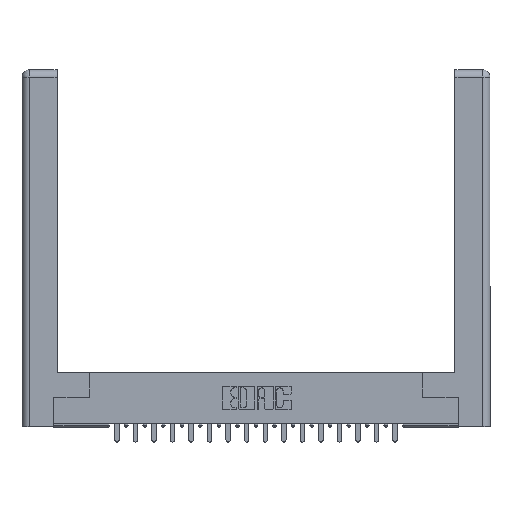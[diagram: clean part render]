
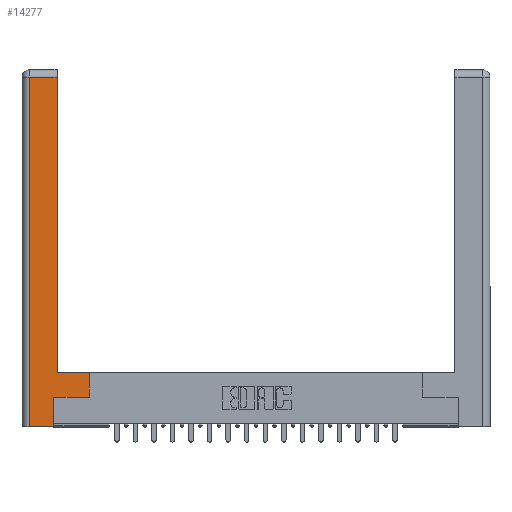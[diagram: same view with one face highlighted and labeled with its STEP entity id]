
A CAD part, top view. The second image highlights one B-rep face of the part: STEP entity #14277.
In plain terms, the highlighted planar face has unit normal (0, 0, 1).
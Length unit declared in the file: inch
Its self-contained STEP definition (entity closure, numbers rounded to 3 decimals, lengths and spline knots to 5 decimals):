
#419 = CARTESIAN_POINT ( 'NONE',  ( 0.265, 0.245, 0. ) ) ;
#942 = CARTESIAN_POINT ( 'NONE',  ( 0.565, 0.245, 0. ) ) ;
#1356 = EDGE_CURVE ( 'NONE', #6592, #10482, #18992, .T. ) ;
#1846 = CARTESIAN_POINT ( 'NONE',  ( 0.265, 0.245, 0. ) ) ;
#2085 = EDGE_CURVE ( 'NONE', #10482, #19898, #3635, .T. ) ;
#2226 = CARTESIAN_POINT ( 'NONE',  ( 0.295, 2.94, 0. ) ) ;
#2466 = ORIENTED_EDGE ( 'NONE', *, *, #19151, .T. ) ;
#2553 = VECTOR ( 'NONE', #2836, 39.37008 ) ;
#2600 = EDGE_CURVE ( 'NONE', #12772, #19252, #6533, .T. ) ;
#2634 = VECTOR ( 'NONE', #10267, 39.37008 ) ;
#2836 = DIRECTION ( 'NONE',  ( 1., 0., 0. ) ) ;
#3635 = LINE ( 'NONE', #16528, #2634 ) ;
#3648 = LINE ( 'NONE', #1846, #16045 ) ;
#4353 = VECTOR ( 'NONE', #9282, 39.37008 ) ;
#4514 = CARTESIAN_POINT ( 'NONE',  ( 0.295, 0.45, 0. ) ) ;
#4773 = DIRECTION ( 'NONE',  ( -1., 0., 0. ) ) ;
#4805 = ORIENTED_EDGE ( 'NONE', *, *, #6696, .T. ) ;
#5311 = ORIENTED_EDGE ( 'NONE', *, *, #2085, .T. ) ;
#6245 = DIRECTION ( 'NONE',  ( 0., 0., -1. ) ) ;
#6289 = EDGE_CURVE ( 'NONE', #19252, #18344, #16684, .T. ) ;
#6533 = LINE ( 'NONE', #16252, #16483 ) ;
#6592 = VERTEX_POINT ( 'NONE', #13665 ) ;
#6696 = EDGE_CURVE ( 'NONE', #19898, #12772, #10075, .T. ) ;
#7159 = AXIS2_PLACEMENT_3D ( 'NONE', #20623, #6245, #4773 ) ;
#7782 = ORIENTED_EDGE ( 'NONE', *, *, #1356, .T. ) ;
#8035 = VECTOR ( 'NONE', #19805, 39.37008 ) ;
#8288 = EDGE_LOOP ( 'NONE', ( #5311, #4805, #14075, #15988, #15586, #17774, #2466, #7782 ) ) ;
#9183 = LINE ( 'NONE', #942, #4353 ) ;
#9282 = DIRECTION ( 'NONE',  ( 1., 0., 0. ) ) ;
#9306 = PLANE ( 'NONE',  #7159 ) ;
#9372 = DIRECTION ( 'NONE',  ( -1., 0., 0. ) ) ;
#9645 = EDGE_CURVE ( 'NONE', #10732, #18544, #9183, .T. ) ;
#10075 = LINE ( 'NONE', #11977, #8035 ) ;
#10267 = DIRECTION ( 'NONE',  ( 0., 1., 0. ) ) ;
#10482 = VERTEX_POINT ( 'NONE', #12575 ) ;
#10528 = DIRECTION ( 'NONE',  ( 0., 1., 0. ) ) ;
#10629 = LINE ( 'NONE', #13599, #19137 ) ;
#10732 = VERTEX_POINT ( 'NONE', #419 ) ;
#10958 = DIRECTION ( 'NONE',  ( 0., -1., 0. ) ) ;
#11651 = VECTOR ( 'NONE', #9372, 39.37008 ) ;
#11977 = CARTESIAN_POINT ( 'NONE',  ( 0.0615, 2.94, 0. ) ) ;
#12575 = CARTESIAN_POINT ( 'NONE',  ( 0.295, 0.45, 0. ) ) ;
#12667 = CARTESIAN_POINT ( 'NONE',  ( 0.565, 0.245, 0. ) ) ;
#12772 = VERTEX_POINT ( 'NONE', #15934 ) ;
#13599 = CARTESIAN_POINT ( 'NONE',  ( 0.565, 0.45, 0. ) ) ;
#13665 = CARTESIAN_POINT ( 'NONE',  ( 0.565, 0.45, 0. ) ) ;
#13752 = CARTESIAN_POINT ( 'NONE',  ( 0.265, 0., 0. ) ) ;
#14075 = ORIENTED_EDGE ( 'NONE', *, *, #2600, .T. ) ;
#14277 = ADVANCED_FACE ( 'NONE', ( #19041 ), #9306, .F. ) ;
#15192 = CARTESIAN_POINT ( 'NONE',  ( 0.0615, 0., 0. ) ) ;
#15586 = ORIENTED_EDGE ( 'NONE', *, *, #17896, .T. ) ;
#15934 = CARTESIAN_POINT ( 'NONE',  ( 0.0615, 2.94, 0. ) ) ;
#15988 = ORIENTED_EDGE ( 'NONE', *, *, #6289, .T. ) ;
#16045 = VECTOR ( 'NONE', #19704, 39.37008 ) ;
#16252 = CARTESIAN_POINT ( 'NONE',  ( 0.0615, 0., 0. ) ) ;
#16483 = VECTOR ( 'NONE', #10958, 39.37008 ) ;
#16528 = CARTESIAN_POINT ( 'NONE',  ( 0.295, 3., 0. ) ) ;
#16684 = LINE ( 'NONE', #17001, #2553 ) ;
#17001 = CARTESIAN_POINT ( 'NONE',  ( 0.265, 0., 0. ) ) ;
#17774 = ORIENTED_EDGE ( 'NONE', *, *, #9645, .T. ) ;
#17896 = EDGE_CURVE ( 'NONE', #18344, #10732, #3648, .T. ) ;
#18344 = VERTEX_POINT ( 'NONE', #13752 ) ;
#18544 = VERTEX_POINT ( 'NONE', #12667 ) ;
#18992 = LINE ( 'NONE', #4514, #11651 ) ;
#19041 = FACE_OUTER_BOUND ( 'NONE', #8288, .T. ) ;
#19137 = VECTOR ( 'NONE', #10528, 39.37008 ) ;
#19151 = EDGE_CURVE ( 'NONE', #18544, #6592, #10629, .T. ) ;
#19252 = VERTEX_POINT ( 'NONE', #15192 ) ;
#19704 = DIRECTION ( 'NONE',  ( 0., 1., 0. ) ) ;
#19805 = DIRECTION ( 'NONE',  ( -1., 0., 0. ) ) ;
#19898 = VERTEX_POINT ( 'NONE', #2226 ) ;
#20623 = CARTESIAN_POINT ( 'NONE',  ( 0., 0., 0. ) ) ;
